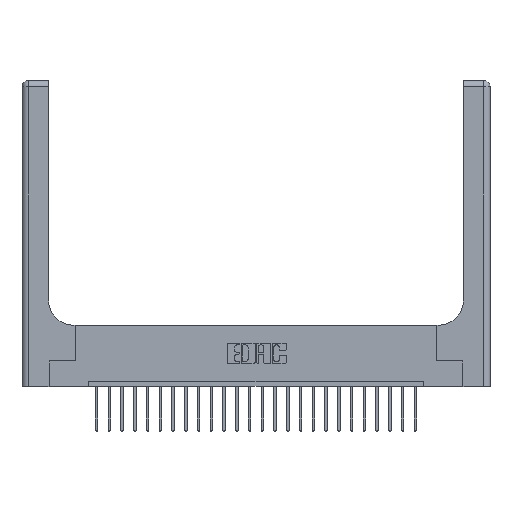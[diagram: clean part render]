
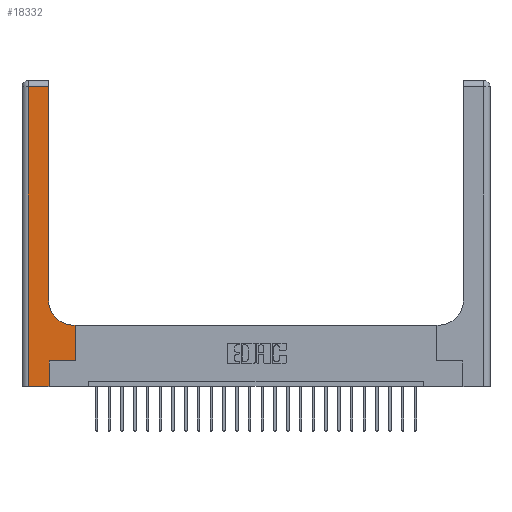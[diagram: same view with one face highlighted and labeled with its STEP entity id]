
A CAD part, top view. The second image highlights one B-rep face of the part: STEP entity #18332.
In plain terms, the highlighted planar face has unit normal (0, 0, 1).
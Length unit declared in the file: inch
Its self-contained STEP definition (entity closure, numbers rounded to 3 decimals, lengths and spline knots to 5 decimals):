
#41 = VERTEX_POINT ( 'NONE', #16250 ) ;
#1283 = DIRECTION ( 'NONE',  ( -1., 0., 0. ) ) ;
#1478 = DIRECTION ( 'NONE',  ( 0., 1., 0. ) ) ;
#1843 = CARTESIAN_POINT ( 'NONE',  ( 0.528, 0.25, 0.37 ) ) ;
#1931 = EDGE_CURVE ( 'NONE', #9695, #3729, #10594, .T. ) ;
#2150 = EDGE_CURVE ( 'NONE', #19231, #9695, #17078, .T. ) ;
#2274 = VECTOR ( 'NONE', #4678, 39.37008 ) ;
#2337 = AXIS2_PLACEMENT_3D ( 'NONE', #12494, #16118, #21051 ) ;
#2440 = VECTOR ( 'NONE', #1283, 39.37008 ) ;
#2459 = VECTOR ( 'NONE', #1478, 39.37008 ) ;
#2590 = ORIENTED_EDGE ( 'NONE', *, *, #13981, .T. ) ;
#2777 = CARTESIAN_POINT ( 'NONE',  ( 0., 2.94, 0.37 ) ) ;
#3274 = VERTEX_POINT ( 'NONE', #5733 ) ;
#3422 = LINE ( 'NONE', #2777, #2274 ) ;
#3729 = VERTEX_POINT ( 'NONE', #7941 ) ;
#4222 = LINE ( 'NONE', #1843, #9653 ) ;
#4678 = DIRECTION ( 'NONE',  ( -1., 0., 0. ) ) ;
#4702 = CARTESIAN_POINT ( 'NONE',  ( 0.265, 0.25, 0.37 ) ) ;
#5292 = LINE ( 'NONE', #21365, #2459 ) ;
#5573 = ORIENTED_EDGE ( 'NONE', *, *, #1931, .T. ) ;
#5733 = CARTESIAN_POINT ( 'NONE',  ( 0.51, 0.6, 0.37 ) ) ;
#7004 = ORIENTED_EDGE ( 'NONE', *, *, #13156, .T. ) ;
#7374 = ORIENTED_EDGE ( 'NONE', *, *, #21351, .T. ) ;
#7843 = EDGE_CURVE ( 'NONE', #14229, #41, #4222, .T. ) ;
#7941 = CARTESIAN_POINT ( 'NONE',  ( 0.265, 0., 0.37 ) ) ;
#8267 = CARTESIAN_POINT ( 'NONE',  ( 0.26, 0.6, 0.37 ) ) ;
#8288 = DIRECTION ( 'NONE',  ( 0., 0., -1. ) ) ;
#8343 = AXIS2_PLACEMENT_3D ( 'NONE', #11844, #8288, #13564 ) ;
#8548 = VERTEX_POINT ( 'NONE', #4702 ) ;
#8666 = ORIENTED_EDGE ( 'NONE', *, *, #17307, .T. ) ;
#8870 = CARTESIAN_POINT ( 'NONE',  ( 0.26, 2.94, 0.37 ) ) ;
#8877 = DIRECTION ( 'NONE',  ( 0., 1., 0. ) ) ;
#9425 = VECTOR ( 'NONE', #8877, 39.37008 ) ;
#9653 = VECTOR ( 'NONE', #21947, 39.37008 ) ;
#9695 = VERTEX_POINT ( 'NONE', #21693 ) ;
#10061 = CARTESIAN_POINT ( 'NONE',  ( 0.528, 0.25, 0.37 ) ) ;
#10594 = LINE ( 'NONE', #22966, #17649 ) ;
#10918 = DIRECTION ( 'NONE',  ( 1., 0., 0. ) ) ;
#11844 = CARTESIAN_POINT ( 'NONE',  ( 0.51, 0.85, 0.37 ) ) ;
#12045 = FACE_OUTER_BOUND ( 'NONE', #18331, .T. ) ;
#12332 = CARTESIAN_POINT ( 'NONE',  ( 0.06, 2.94, 0.37 ) ) ;
#12494 = CARTESIAN_POINT ( 'NONE',  ( 0., 3., 0.37 ) ) ;
#13156 = EDGE_CURVE ( 'NONE', #3729, #8548, #13954, .T. ) ;
#13564 = DIRECTION ( 'NONE',  ( 1., 0., 0. ) ) ;
#13954 = LINE ( 'NONE', #23372, #9425 ) ;
#13981 = EDGE_CURVE ( 'NONE', #8548, #14229, #19020, .T. ) ;
#14094 = LINE ( 'NONE', #8267, #2440 ) ;
#14229 = VERTEX_POINT ( 'NONE', #10061 ) ;
#14356 = PLANE ( 'NONE',  #2337 ) ;
#14800 = ORIENTED_EDGE ( 'NONE', *, *, #16397, .T. ) ;
#15282 = ORIENTED_EDGE ( 'NONE', *, *, #7843, .T. ) ;
#15740 = DIRECTION ( 'NONE',  ( 1., 0., 0. ) ) ;
#16118 = DIRECTION ( 'NONE',  ( 0., 0., -1. ) ) ;
#16133 = ORIENTED_EDGE ( 'NONE', *, *, #2150, .T. ) ;
#16235 = VECTOR ( 'NONE', #21915, 39.37008 ) ;
#16250 = CARTESIAN_POINT ( 'NONE',  ( 0.528, 0.6, 0.37 ) ) ;
#16397 = EDGE_CURVE ( 'NONE', #22204, #17363, #5292, .T. ) ;
#17078 = LINE ( 'NONE', #22159, #16235 ) ;
#17307 = EDGE_CURVE ( 'NONE', #41, #3274, #14094, .T. ) ;
#17363 = VERTEX_POINT ( 'NONE', #8870 ) ;
#17649 = VECTOR ( 'NONE', #15740, 39.37008 ) ;
#17856 = VECTOR ( 'NONE', #10918, 39.37008 ) ;
#18331 = EDGE_LOOP ( 'NONE', ( #14800, #7374, #16133, #5573, #7004, #2590, #15282, #8666, #18510 ) ) ;
#18332 = ADVANCED_FACE ( 'NONE', ( #12045 ), #14356, .F. ) ;
#18510 = ORIENTED_EDGE ( 'NONE', *, *, #23439, .T. ) ;
#19020 = LINE ( 'NONE', #21855, #17856 ) ;
#19231 = VERTEX_POINT ( 'NONE', #12332 ) ;
#21051 = DIRECTION ( 'NONE',  ( -1., 0., 0. ) ) ;
#21351 = EDGE_CURVE ( 'NONE', #17363, #19231, #3422, .T. ) ;
#21365 = CARTESIAN_POINT ( 'NONE',  ( 0.26, 3., 0.37 ) ) ;
#21693 = CARTESIAN_POINT ( 'NONE',  ( 0.06, 0., 0.37 ) ) ;
#21855 = CARTESIAN_POINT ( 'NONE',  ( 0.265, 0.25, 0.37 ) ) ;
#21915 = DIRECTION ( 'NONE',  ( 0., -1., 0. ) ) ;
#21947 = DIRECTION ( 'NONE',  ( 0., 1., 0. ) ) ;
#22159 = CARTESIAN_POINT ( 'NONE',  ( 0.06, 3., 0.37 ) ) ;
#22204 = VERTEX_POINT ( 'NONE', #22591 ) ;
#22591 = CARTESIAN_POINT ( 'NONE',  ( 0.26, 0.85, 0.37 ) ) ;
#22864 = CIRCLE ( 'NONE', #8343, 0.25 ) ;
#22966 = CARTESIAN_POINT ( 'NONE',  ( 0., 0., 0.37 ) ) ;
#23372 = CARTESIAN_POINT ( 'NONE',  ( 0.265, 0., 0.37 ) ) ;
#23439 = EDGE_CURVE ( 'NONE', #3274, #22204, #22864, .T. ) ;
